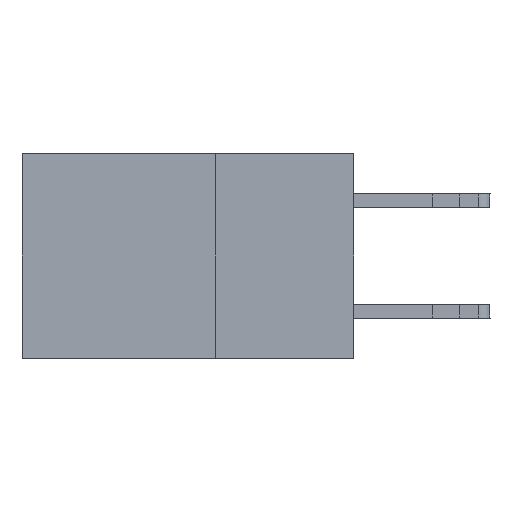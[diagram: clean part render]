
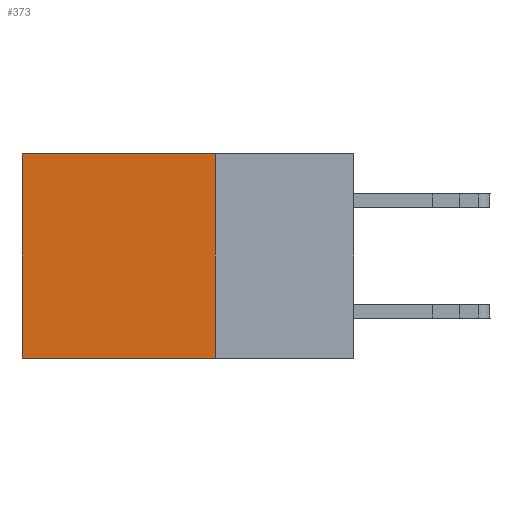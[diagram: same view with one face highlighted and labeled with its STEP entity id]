
A CAD part, left-side view. The second image highlights one B-rep face of the part: STEP entity #373.
In plain terms, the highlighted planar face has unit normal (-1, 0, 0).
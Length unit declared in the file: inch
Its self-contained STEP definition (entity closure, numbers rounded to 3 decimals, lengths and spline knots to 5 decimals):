
#373 = ADVANCED_FACE ( 'NONE', ( #6494 ), #27849, .F. ) ;
#431 = CARTESIAN_POINT ( 'NONE',  ( 0.2875, 0.25, 0. ) ) ;
#1466 = VERTEX_POINT ( 'NONE', #17949 ) ;
#1543 = LINE ( 'NONE', #3986, #17052 ) ;
#1565 = ORIENTED_EDGE ( 'NONE', *, *, #15733, .F. ) ;
#3986 = CARTESIAN_POINT ( 'NONE',  ( 0.2875, 0.25, -0.37 ) ) ;
#4699 = ORIENTED_EDGE ( 'NONE', *, *, #18008, .T. ) ;
#5009 = VERTEX_POINT ( 'NONE', #8720 ) ;
#5648 = DIRECTION ( 'NONE',  ( 0., 1., 0. ) ) ;
#6344 = DIRECTION ( 'NONE',  ( 0., 0., -1. ) ) ;
#6439 = DIRECTION ( 'NONE',  ( 0., 1., 0. ) ) ;
#6494 = FACE_OUTER_BOUND ( 'NONE', #11827, .T. ) ;
#6807 = CARTESIAN_POINT ( 'NONE',  ( 0.2875, 0.25, -0.37 ) ) ;
#8720 = CARTESIAN_POINT ( 'NONE',  ( 0.2875, 0.6, 0. ) ) ;
#9134 = VECTOR ( 'NONE', #13851, 39.37008 ) ;
#11070 = CARTESIAN_POINT ( 'NONE',  ( 0.2875, 0.25, 0. ) ) ;
#11416 = LINE ( 'NONE', #11070, #33432 ) ;
#11827 = EDGE_LOOP ( 'NONE', ( #13530, #1565, #19793, #4699 ) ) ;
#11917 = DIRECTION ( 'NONE',  ( 1., 0., 0. ) ) ;
#12855 = LINE ( 'NONE', #431, #27009 ) ;
#13272 = EDGE_CURVE ( 'NONE', #22570, #19969, #12855, .T. ) ;
#13530 = ORIENTED_EDGE ( 'NONE', *, *, #13710, .T. ) ;
#13710 = EDGE_CURVE ( 'NONE', #5009, #1466, #23867, .T. ) ;
#13851 = DIRECTION ( 'NONE',  ( 0., 0., -1. ) ) ;
#15733 = EDGE_CURVE ( 'NONE', #19969, #1466, #1543, .T. ) ;
#17052 = VECTOR ( 'NONE', #6439, 39.37008 ) ;
#17511 = CARTESIAN_POINT ( 'NONE',  ( 0.2875, 0.25, 0. ) ) ;
#17949 = CARTESIAN_POINT ( 'NONE',  ( 0.2875, 0.6, -0.37 ) ) ;
#18008 = EDGE_CURVE ( 'NONE', #22570, #5009, #11416, .T. ) ;
#19793 = ORIENTED_EDGE ( 'NONE', *, *, #13272, .F. ) ;
#19909 = AXIS2_PLACEMENT_3D ( 'NONE', #17511, #11917, #23119 ) ;
#19969 = VERTEX_POINT ( 'NONE', #6807 ) ;
#21897 = CARTESIAN_POINT ( 'NONE',  ( 0.2875, 0.6, 0. ) ) ;
#22570 = VERTEX_POINT ( 'NONE', #25296 ) ;
#23119 = DIRECTION ( 'NONE',  ( 0., 0., -1. ) ) ;
#23867 = LINE ( 'NONE', #21897, #9134 ) ;
#25296 = CARTESIAN_POINT ( 'NONE',  ( 0.2875, 0.25, 0. ) ) ;
#27009 = VECTOR ( 'NONE', #6344, 39.37008 ) ;
#27849 = PLANE ( 'NONE',  #19909 ) ;
#33432 = VECTOR ( 'NONE', #5648, 39.37008 ) ;
